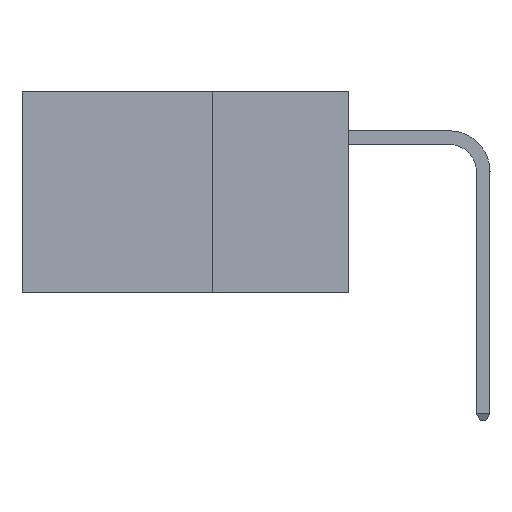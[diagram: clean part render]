
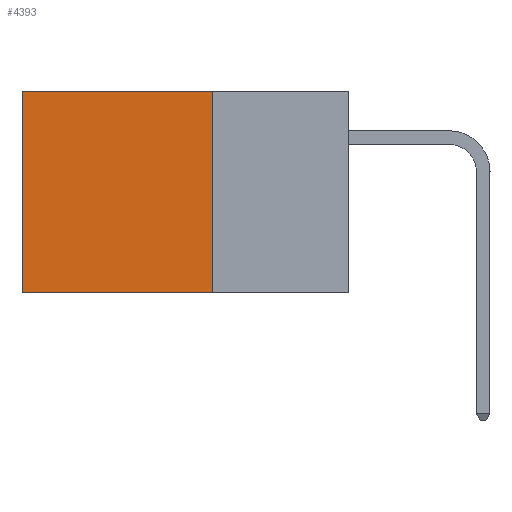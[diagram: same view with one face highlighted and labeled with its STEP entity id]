
A CAD part, left-side view. The second image highlights one B-rep face of the part: STEP entity #4393.
In plain terms, the highlighted planar face has unit normal (-1, 0, 0).
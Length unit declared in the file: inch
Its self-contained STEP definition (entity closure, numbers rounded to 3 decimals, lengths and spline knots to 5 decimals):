
#669 = EDGE_CURVE ( 'NONE', #15980, #7430, #3498, .T. ) ;
#1088 = EDGE_LOOP ( 'NONE', ( #14702, #2459, #7310, #7563 ) ) ;
#1822 = VECTOR ( 'NONE', #9919, 39.37008 ) ;
#1845 = LINE ( 'NONE', #14493, #15846 ) ;
#1860 = DIRECTION ( 'NONE',  ( 0., 1., 0. ) ) ;
#2108 = DIRECTION ( 'NONE',  ( 0., 0., -1. ) ) ;
#2301 = EDGE_CURVE ( 'NONE', #7430, #16155, #1845, .T. ) ;
#2459 = ORIENTED_EDGE ( 'NONE', *, *, #2301, .F. ) ;
#3151 = CARTESIAN_POINT ( 'NONE',  ( 0.2875, 0.25, 0. ) ) ;
#3232 = FACE_OUTER_BOUND ( 'NONE', #1088, .T. ) ;
#3498 = LINE ( 'NONE', #12203, #1822 ) ;
#3971 = CARTESIAN_POINT ( 'NONE',  ( 0.2875, 0.25, 0. ) ) ;
#4393 = ADVANCED_FACE ( 'NONE', ( #3232 ), #14704, .F. ) ;
#4738 = AXIS2_PLACEMENT_3D ( 'NONE', #3151, #8293, #12531 ) ;
#5665 = CARTESIAN_POINT ( 'NONE',  ( 0.2875, 0.6, 0. ) ) ;
#7310 = ORIENTED_EDGE ( 'NONE', *, *, #669, .F. ) ;
#7430 = VERTEX_POINT ( 'NONE', #14094 ) ;
#7563 = ORIENTED_EDGE ( 'NONE', *, *, #16017, .T. ) ;
#8293 = DIRECTION ( 'NONE',  ( 1., 0., 0. ) ) ;
#8372 = VECTOR ( 'NONE', #1860, 39.37008 ) ;
#8518 = LINE ( 'NONE', #13666, #10841 ) ;
#9439 = VERTEX_POINT ( 'NONE', #5665 ) ;
#9789 = CARTESIAN_POINT ( 'NONE',  ( 0.2875, 0.6, -0.37 ) ) ;
#9919 = DIRECTION ( 'NONE',  ( 0., 0., -1. ) ) ;
#10841 = VECTOR ( 'NONE', #2108, 39.37008 ) ;
#11812 = EDGE_CURVE ( 'NONE', #9439, #16155, #8518, .T. ) ;
#12203 = CARTESIAN_POINT ( 'NONE',  ( 0.2875, 0.25, 0. ) ) ;
#12531 = DIRECTION ( 'NONE',  ( 0., 0., -1. ) ) ;
#13225 = DIRECTION ( 'NONE',  ( 0., 1., 0. ) ) ;
#13666 = CARTESIAN_POINT ( 'NONE',  ( 0.2875, 0.6, 0. ) ) ;
#14094 = CARTESIAN_POINT ( 'NONE',  ( 0.2875, 0.25, -0.37 ) ) ;
#14271 = LINE ( 'NONE', #3971, #8372 ) ;
#14493 = CARTESIAN_POINT ( 'NONE',  ( 0.2875, 0.25, -0.37 ) ) ;
#14702 = ORIENTED_EDGE ( 'NONE', *, *, #11812, .T. ) ;
#14704 = PLANE ( 'NONE',  #4738 ) ;
#15542 = CARTESIAN_POINT ( 'NONE',  ( 0.2875, 0.25, 0. ) ) ;
#15846 = VECTOR ( 'NONE', #13225, 39.37008 ) ;
#15980 = VERTEX_POINT ( 'NONE', #15542 ) ;
#16017 = EDGE_CURVE ( 'NONE', #15980, #9439, #14271, .T. ) ;
#16155 = VERTEX_POINT ( 'NONE', #9789 ) ;
